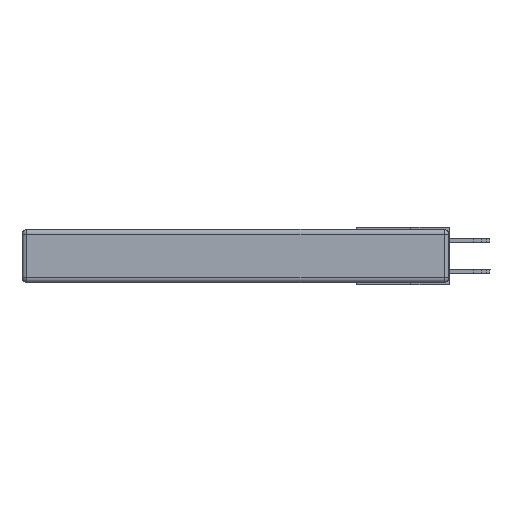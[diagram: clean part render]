
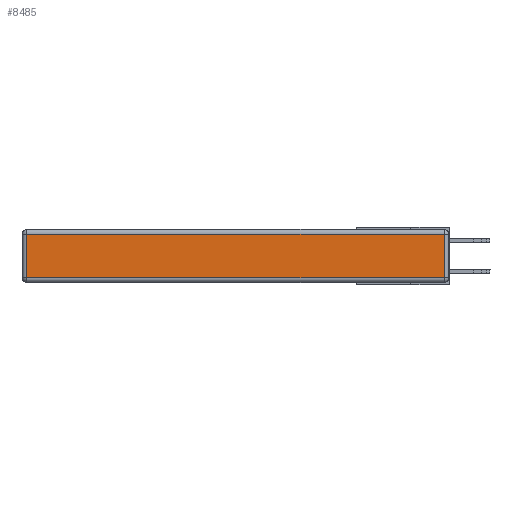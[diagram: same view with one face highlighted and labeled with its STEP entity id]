
A CAD part, left-side view. The second image highlights one B-rep face of the part: STEP entity #8485.
In plain terms, the highlighted planar face has unit normal (-1, 0, 0).
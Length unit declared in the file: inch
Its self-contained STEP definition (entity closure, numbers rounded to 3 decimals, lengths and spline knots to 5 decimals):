
#298 = VERTEX_POINT ( 'NONE', #16350 ) ;
#1398 = EDGE_CURVE ( 'NONE', #26616, #15981, #5289, .T. ) ;
#1434 = LINE ( 'NONE', #6050, #17357 ) ;
#1806 = CARTESIAN_POINT ( 'NONE',  ( 0., 0.03, -0.313 ) ) ;
#3034 = CARTESIAN_POINT ( 'NONE',  ( 0., 0., -0.313 ) ) ;
#3290 = PLANE ( 'NONE',  #26712 ) ;
#3392 = DIRECTION ( 'NONE',  ( 0., 0., 1. ) ) ;
#5289 = LINE ( 'NONE', #7672, #25738 ) ;
#5392 = DIRECTION ( 'NONE',  ( -1., 0., 0. ) ) ;
#6050 = CARTESIAN_POINT ( 'NONE',  ( 0., 2.72, -0.343 ) ) ;
#7301 = VECTOR ( 'NONE', #24067, 39.37008 ) ;
#7672 = CARTESIAN_POINT ( 'NONE',  ( 0., 0.03, -0.343 ) ) ;
#8485 = ADVANCED_FACE ( 'NONE', ( #22712 ), #3290, .T. ) ;
#11590 = ORIENTED_EDGE ( 'NONE', *, *, #1398, .T. ) ;
#11893 = CARTESIAN_POINT ( 'NONE',  ( 0., 2.72, -0.03 ) ) ;
#12461 = EDGE_CURVE ( 'NONE', #21924, #298, #1434, .T. ) ;
#14489 = ORIENTED_EDGE ( 'NONE', *, *, #20833, .T. ) ;
#15981 = VERTEX_POINT ( 'NONE', #22945 ) ;
#16350 = CARTESIAN_POINT ( 'NONE',  ( 0., 2.72, -0.313 ) ) ;
#17357 = VECTOR ( 'NONE', #20784, 39.37008 ) ;
#17726 = DIRECTION ( 'NONE',  ( 0., 0., 1. ) ) ;
#18506 = EDGE_CURVE ( 'NONE', #298, #26616, #19627, .T. ) ;
#19627 = LINE ( 'NONE', #3034, #7301 ) ;
#20623 = ORIENTED_EDGE ( 'NONE', *, *, #12461, .T. ) ;
#20784 = DIRECTION ( 'NONE',  ( 0., 0., -1. ) ) ;
#20833 = EDGE_CURVE ( 'NONE', #15981, #21924, #22765, .T. ) ;
#21469 = CARTESIAN_POINT ( 'NONE',  ( 0., 2.75, -0.03 ) ) ;
#21924 = VERTEX_POINT ( 'NONE', #11893 ) ;
#22712 = FACE_OUTER_BOUND ( 'NONE', #23935, .T. ) ;
#22765 = LINE ( 'NONE', #21469, #23409 ) ;
#22945 = CARTESIAN_POINT ( 'NONE',  ( 0., 0.03, -0.03 ) ) ;
#23289 = ORIENTED_EDGE ( 'NONE', *, *, #18506, .T. ) ;
#23409 = VECTOR ( 'NONE', #25289, 39.37008 ) ;
#23935 = EDGE_LOOP ( 'NONE', ( #23289, #11590, #14489, #20623 ) ) ;
#24067 = DIRECTION ( 'NONE',  ( 0., -1., 0. ) ) ;
#25289 = DIRECTION ( 'NONE',  ( 0., 1., 0. ) ) ;
#25738 = VECTOR ( 'NONE', #3392, 39.37008 ) ;
#25970 = CARTESIAN_POINT ( 'NONE',  ( 0., 0., -0.343 ) ) ;
#26616 = VERTEX_POINT ( 'NONE', #1806 ) ;
#26712 = AXIS2_PLACEMENT_3D ( 'NONE', #25970, #5392, #17726 ) ;
